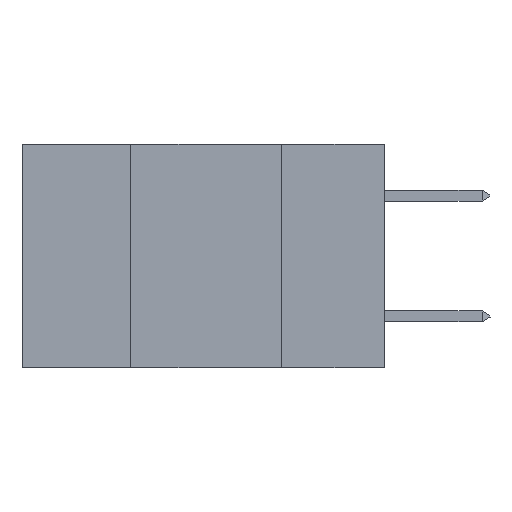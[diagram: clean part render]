
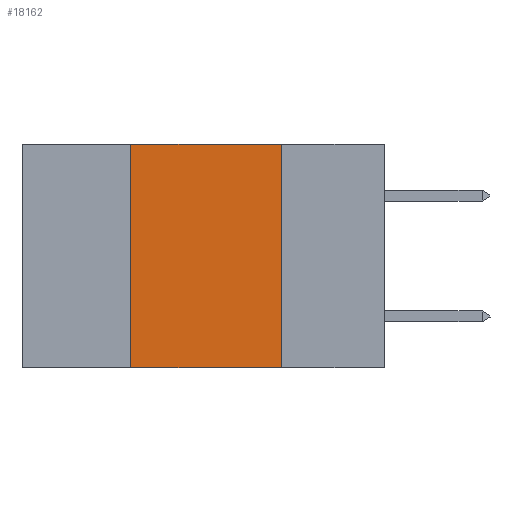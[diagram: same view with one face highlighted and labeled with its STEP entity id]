
A CAD part, left-side view. The second image highlights one B-rep face of the part: STEP entity #18162.
In plain terms, the highlighted planar face has unit normal (-1, 0, 0).
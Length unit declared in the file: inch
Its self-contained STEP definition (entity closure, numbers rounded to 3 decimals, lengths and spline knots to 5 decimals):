
#93 = VERTEX_POINT ( 'NONE', #22763 ) ;
#556 = DIRECTION ( 'NONE',  ( 0., -1., 0. ) ) ;
#795 = CARTESIAN_POINT ( 'NONE',  ( 0., 0.6, -0.37 ) ) ;
#929 = LINE ( 'NONE', #12420, #19685 ) ;
#1422 = ORIENTED_EDGE ( 'NONE', *, *, #3860, .T. ) ;
#2293 = LINE ( 'NONE', #17761, #10997 ) ;
#3016 = ORIENTED_EDGE ( 'NONE', *, *, #13623, .F. ) ;
#3164 = VERTEX_POINT ( 'NONE', #10906 ) ;
#3860 = EDGE_CURVE ( 'NONE', #17755, #3164, #14435, .T. ) ;
#4658 = VECTOR ( 'NONE', #556, 39.37008 ) ;
#4812 = ORIENTED_EDGE ( 'NONE', *, *, #10092, .F. ) ;
#4817 = PLANE ( 'NONE',  #22046 ) ;
#6983 = CARTESIAN_POINT ( 'NONE',  ( 0., 0.6, 0. ) ) ;
#7023 = DIRECTION ( 'NONE',  ( 0., 0., -1. ) ) ;
#7976 = EDGE_LOOP ( 'NONE', ( #4812, #18029, #3016, #1422 ) ) ;
#8963 = LINE ( 'NONE', #6983, #13819 ) ;
#10092 = EDGE_CURVE ( 'NONE', #93, #3164, #2293, .T. ) ;
#10428 = DIRECTION ( 'NONE',  ( 0., 0., -1. ) ) ;
#10526 = CARTESIAN_POINT ( 'NONE',  ( 0., 0.42, -0.37 ) ) ;
#10906 = CARTESIAN_POINT ( 'NONE',  ( 0., 0.17, -0.37 ) ) ;
#10997 = VECTOR ( 'NONE', #7023, 39.37008 ) ;
#12420 = CARTESIAN_POINT ( 'NONE',  ( 0., 0.42, 0. ) ) ;
#12464 = CARTESIAN_POINT ( 'NONE',  ( 0., 0.42, 0. ) ) ;
#13623 = EDGE_CURVE ( 'NONE', #17755, #21861, #929, .T. ) ;
#13819 = VECTOR ( 'NONE', #19543, 39.37008 ) ;
#14435 = LINE ( 'NONE', #795, #4658 ) ;
#16051 = DIRECTION ( 'NONE',  ( 0., 0., 1. ) ) ;
#17450 = CARTESIAN_POINT ( 'NONE',  ( 0., 0.6, 0. ) ) ;
#17755 = VERTEX_POINT ( 'NONE', #10526 ) ;
#17761 = CARTESIAN_POINT ( 'NONE',  ( 0., 0.17, 0. ) ) ;
#18029 = ORIENTED_EDGE ( 'NONE', *, *, #18893, .F. ) ;
#18162 = ADVANCED_FACE ( 'NONE', ( #20960 ), #4817, .F. ) ;
#18893 = EDGE_CURVE ( 'NONE', #21861, #93, #8963, .T. ) ;
#19543 = DIRECTION ( 'NONE',  ( 0., -1., 0. ) ) ;
#19685 = VECTOR ( 'NONE', #16051, 39.37008 ) ;
#20960 = FACE_OUTER_BOUND ( 'NONE', #7976, .T. ) ;
#21001 = DIRECTION ( 'NONE',  ( 1., 0., 0. ) ) ;
#21861 = VERTEX_POINT ( 'NONE', #12464 ) ;
#22046 = AXIS2_PLACEMENT_3D ( 'NONE', #17450, #21001, #10428 ) ;
#22763 = CARTESIAN_POINT ( 'NONE',  ( 0., 0.17, 0. ) ) ;
